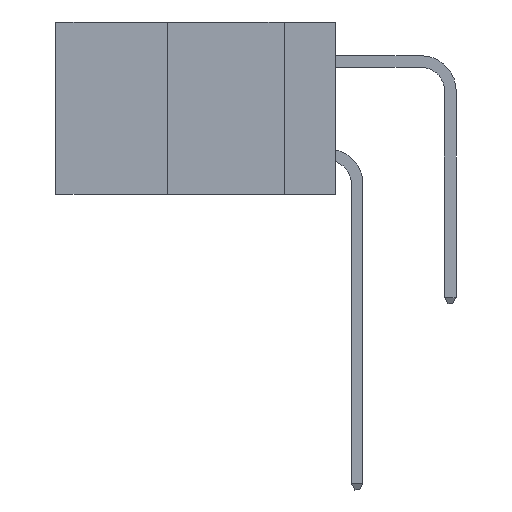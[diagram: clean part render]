
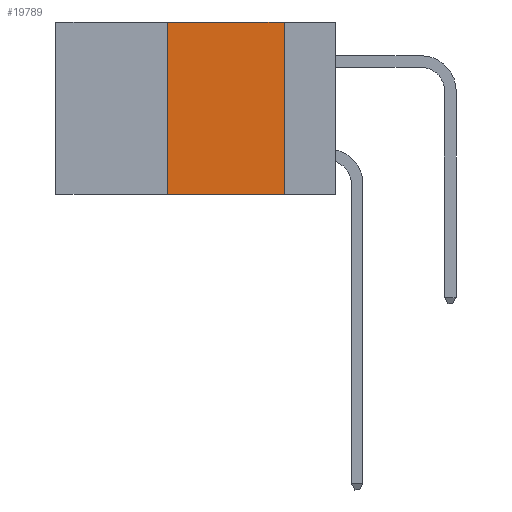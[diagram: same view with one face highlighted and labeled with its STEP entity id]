
A CAD part, left-side view. The second image highlights one B-rep face of the part: STEP entity #19789.
In plain terms, the highlighted planar face has unit normal (-1, 0, 0).
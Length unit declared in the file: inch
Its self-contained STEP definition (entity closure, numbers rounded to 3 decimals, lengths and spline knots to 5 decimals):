
#1527 = ORIENTED_EDGE ( 'NONE', *, *, #2247, .T. ) ;
#1851 = CARTESIAN_POINT ( 'NONE',  ( 0., 0.36, 0. ) ) ;
#2247 = EDGE_CURVE ( 'NONE', #8008, #16054, #7251, .T. ) ;
#3593 = DIRECTION ( 'NONE',  ( 0., 0., -1. ) ) ;
#3812 = EDGE_CURVE ( 'NONE', #22836, #16054, #11023, .T. ) ;
#4643 = CARTESIAN_POINT ( 'NONE',  ( 0., 0.11, -0.37 ) ) ;
#5447 = DIRECTION ( 'NONE',  ( 0., 0., -1. ) ) ;
#6291 = ORIENTED_EDGE ( 'NONE', *, *, #3812, .F. ) ;
#6907 = EDGE_CURVE ( 'NONE', #8008, #17465, #20907, .T. ) ;
#7251 = LINE ( 'NONE', #10667, #21220 ) ;
#8008 = VERTEX_POINT ( 'NONE', #9302 ) ;
#9302 = CARTESIAN_POINT ( 'NONE',  ( 0., 0.36, -0.37 ) ) ;
#10020 = AXIS2_PLACEMENT_3D ( 'NONE', #22673, #20901, #5447 ) ;
#10667 = CARTESIAN_POINT ( 'NONE',  ( 0., 0.6, -0.37 ) ) ;
#10790 = ORIENTED_EDGE ( 'NONE', *, *, #16923, .F. ) ;
#11023 = LINE ( 'NONE', #24341, #23649 ) ;
#13278 = CARTESIAN_POINT ( 'NONE',  ( 0., 0.36, 0. ) ) ;
#14923 = EDGE_LOOP ( 'NONE', ( #6291, #10790, #24157, #1527 ) ) ;
#14982 = PLANE ( 'NONE',  #10020 ) ;
#16054 = VERTEX_POINT ( 'NONE', #4643 ) ;
#16287 = DIRECTION ( 'NONE',  ( 0., -1., 0. ) ) ;
#16923 = EDGE_CURVE ( 'NONE', #17465, #22836, #19652, .T. ) ;
#17465 = VERTEX_POINT ( 'NONE', #13278 ) ;
#18010 = CARTESIAN_POINT ( 'NONE',  ( 0., 0.6, 0. ) ) ;
#18644 = VECTOR ( 'NONE', #24689, 39.37008 ) ;
#19630 = VECTOR ( 'NONE', #21927, 39.37008 ) ;
#19652 = LINE ( 'NONE', #18010, #19630 ) ;
#19789 = ADVANCED_FACE ( 'NONE', ( #20774 ), #14982, .F. ) ;
#20774 = FACE_OUTER_BOUND ( 'NONE', #14923, .T. ) ;
#20901 = DIRECTION ( 'NONE',  ( 1., 0., 0. ) ) ;
#20907 = LINE ( 'NONE', #1851, #18644 ) ;
#21220 = VECTOR ( 'NONE', #16287, 39.37008 ) ;
#21927 = DIRECTION ( 'NONE',  ( 0., -1., 0. ) ) ;
#22673 = CARTESIAN_POINT ( 'NONE',  ( 0., 0.6, 0. ) ) ;
#22836 = VERTEX_POINT ( 'NONE', #23596 ) ;
#23596 = CARTESIAN_POINT ( 'NONE',  ( 0., 0.11, 0. ) ) ;
#23649 = VECTOR ( 'NONE', #3593, 39.37008 ) ;
#24157 = ORIENTED_EDGE ( 'NONE', *, *, #6907, .F. ) ;
#24341 = CARTESIAN_POINT ( 'NONE',  ( 0., 0.11, 0. ) ) ;
#24689 = DIRECTION ( 'NONE',  ( 0., 0., 1. ) ) ;
